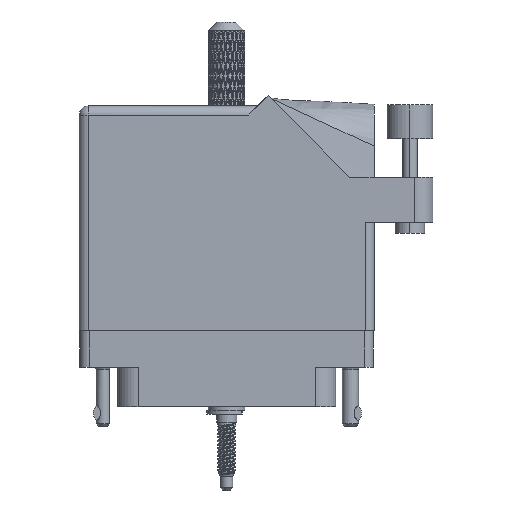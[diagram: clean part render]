
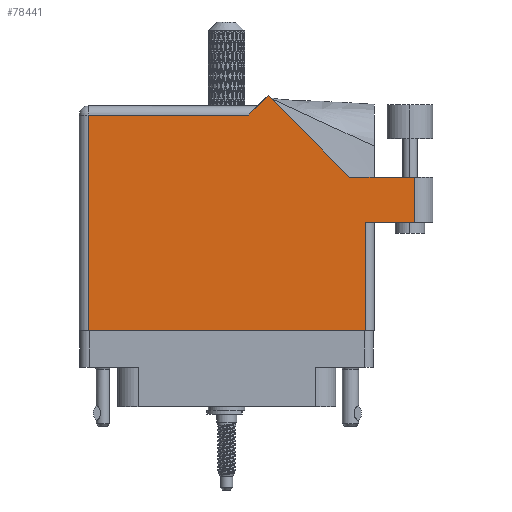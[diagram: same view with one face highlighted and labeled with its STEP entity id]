
A CAD part, front view. The second image highlights one B-rep face of the part: STEP entity #78441.
In plain terms, the highlighted face is planar.
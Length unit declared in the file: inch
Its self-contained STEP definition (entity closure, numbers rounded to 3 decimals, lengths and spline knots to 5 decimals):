
#902 = EDGE_CURVE ( 'NONE', #83423, #99205, #110300, .T. ) ;
#1014 = VECTOR ( 'NONE', #47891, 39.37008 ) ;
#1183 = ORIENTED_EDGE ( 'NONE', *, *, #83351, .T. ) ;
#5595 = EDGE_CURVE ( 'NONE', #93148, #32212, #73731, .T. ) ;
#9262 = VECTOR ( 'NONE', #13915, 39.37008 ) ;
#9729 = FACE_OUTER_BOUND ( 'NONE', #104813, .T. ) ;
#11944 = LINE ( 'NONE', #46448, #24510 ) ;
#12029 = LINE ( 'NONE', #30674, #9262 ) ;
#12429 = LINE ( 'NONE', #108214, #73568 ) ;
#13915 = DIRECTION ( 'NONE',  ( -0.707, -0.707, 0. ) ) ;
#14635 = VECTOR ( 'NONE', #45755, 39.37008 ) ;
#15991 = EDGE_CURVE ( 'NONE', #107716, #38520, #11944, .T. ) ;
#16409 = ORIENTED_EDGE ( 'NONE', *, *, #91203, .T. ) ;
#18614 = VECTOR ( 'NONE', #18669, 39.37008 ) ;
#18669 = DIRECTION ( 'NONE',  ( 0., -1., 0. ) ) ;
#21167 = ORIENTED_EDGE ( 'NONE', *, *, #902, .T. ) ;
#21857 = CARTESIAN_POINT ( 'NONE',  ( 0.943, 0.637, 0.455 ) ) ;
#22376 = CARTESIAN_POINT ( 'NONE',  ( 1.28, 0.637, 0.455 ) ) ;
#24510 = VECTOR ( 'NONE', #65078, 39.37008 ) ;
#29082 = ORIENTED_EDGE ( 'NONE', *, *, #5595, .T. ) ;
#30674 = CARTESIAN_POINT ( 'NONE',  ( 0.212, 1.43, 0.455 ) ) ;
#32212 = VERTEX_POINT ( 'NONE', #22376 ) ;
#37810 = ORIENTED_EDGE ( 'NONE', *, *, #109860, .T. ) ;
#38520 = VERTEX_POINT ( 'NONE', #48944 ) ;
#45755 = DIRECTION ( 'NONE',  ( -1., 0., 0. ) ) ;
#46263 = CARTESIAN_POINT ( 'NONE',  ( -0.943, -0.1, 0.455 ) ) ;
#46448 = CARTESIAN_POINT ( 'NONE',  ( 0.83942, 0.944, 0.455 ) ) ;
#47891 = DIRECTION ( 'NONE',  ( 0., 1., 0. ) ) ;
#48705 = EDGE_CURVE ( 'NONE', #56449, #93148, #69207, .T. ) ;
#48944 = CARTESIAN_POINT ( 'NONE',  ( 0.28271, 1.50071, 0.455 ) ) ;
#51887 = CARTESIAN_POINT ( 'NONE',  ( 0.15, 1.368, 0.455 ) ) ;
#52191 = DIRECTION ( 'NONE',  ( 0., 1., 0. ) ) ;
#55043 = ORIENTED_EDGE ( 'NONE', *, *, #15991, .T. ) ;
#56179 = AXIS2_PLACEMENT_3D ( 'NONE', #99068, #108773, #74246 ) ;
#56449 = VERTEX_POINT ( 'NONE', #102556 ) ;
#65078 = DIRECTION ( 'NONE',  ( -0.707, 0.707, 0. ) ) ;
#68966 = EDGE_CURVE ( 'NONE', #32212, #102187, #104663, .T. ) ;
#69207 = LINE ( 'NONE', #21857, #1014 ) ;
#71980 = CARTESIAN_POINT ( 'NONE',  ( 1.005, 0.637, 0.455 ) ) ;
#73269 = DIRECTION ( 'NONE',  ( -1., 0., 0. ) ) ;
#73568 = VECTOR ( 'NONE', #105772, 39.37008 ) ;
#73731 = LINE ( 'NONE', #71980, #90418 ) ;
#74245 = CARTESIAN_POINT ( 'NONE',  ( 1.28, 0.944, 0.455 ) ) ;
#74246 = DIRECTION ( 'NONE',  ( -1., 0., 0. ) ) ;
#78165 = ORIENTED_EDGE ( 'NONE', *, *, #95701, .T. ) ;
#78441 = ADVANCED_FACE ( 'NONE', ( #9729 ), #108390, .F. ) ;
#80854 = CARTESIAN_POINT ( 'NONE',  ( 0.83942, 0.944, 0.455 ) ) ;
#81831 = CARTESIAN_POINT ( 'NONE',  ( -1.005, 1.368, 0.455 ) ) ;
#82678 = LINE ( 'NONE', #88415, #85456 ) ;
#83351 = EDGE_CURVE ( 'NONE', #96134, #83423, #88320, .T. ) ;
#83423 = VERTEX_POINT ( 'NONE', #98535 ) ;
#85456 = VECTOR ( 'NONE', #73269, 39.37008 ) ;
#86343 = ORIENTED_EDGE ( 'NONE', *, *, #68966, .T. ) ;
#87817 = CARTESIAN_POINT ( 'NONE',  ( -0.943, -0.1, 0.455 ) ) ;
#88320 = LINE ( 'NONE', #81831, #14635 ) ;
#88415 = CARTESIAN_POINT ( 'NONE',  ( 1.405, 0.944, 0.455 ) ) ;
#90148 = CARTESIAN_POINT ( 'NONE',  ( 0.943, 0.637, 0.455 ) ) ;
#90418 = VECTOR ( 'NONE', #106898, 39.37008 ) ;
#91203 = EDGE_CURVE ( 'NONE', #99205, #56449, #12429, .T. ) ;
#93148 = VERTEX_POINT ( 'NONE', #90148 ) ;
#95701 = EDGE_CURVE ( 'NONE', #38520, #96134, #12029, .T. ) ;
#96134 = VERTEX_POINT ( 'NONE', #51887 ) ;
#96307 = VECTOR ( 'NONE', #52191, 39.37008 ) ;
#98535 = CARTESIAN_POINT ( 'NONE',  ( -0.943, 1.368, 0.455 ) ) ;
#99068 = CARTESIAN_POINT ( 'NONE',  ( -1.005, 1.43, 0.455 ) ) ;
#99205 = VERTEX_POINT ( 'NONE', #87817 ) ;
#102187 = VERTEX_POINT ( 'NONE', #74245 ) ;
#102556 = CARTESIAN_POINT ( 'NONE',  ( 0.943, -0.1, 0.455 ) ) ;
#104663 = LINE ( 'NONE', #105329, #96307 ) ;
#104813 = EDGE_LOOP ( 'NONE', ( #29082, #86343, #37810, #55043, #78165, #1183, #21167, #16409, #114657 ) ) ;
#105329 = CARTESIAN_POINT ( 'NONE',  ( 1.28, 0.944, 0.455 ) ) ;
#105772 = DIRECTION ( 'NONE',  ( 1., 0., 0. ) ) ;
#106898 = DIRECTION ( 'NONE',  ( 1., 0., 0. ) ) ;
#107716 = VERTEX_POINT ( 'NONE', #80854 ) ;
#108214 = CARTESIAN_POINT ( 'NONE',  ( -1.005, -0.1, 0.455 ) ) ;
#108390 = PLANE ( 'NONE',  #56179 ) ;
#108773 = DIRECTION ( 'NONE',  ( 0., 0., -1. ) ) ;
#109860 = EDGE_CURVE ( 'NONE', #102187, #107716, #82678, .T. ) ;
#110300 = LINE ( 'NONE', #46263, #18614 ) ;
#114657 = ORIENTED_EDGE ( 'NONE', *, *, #48705, .T. ) ;
